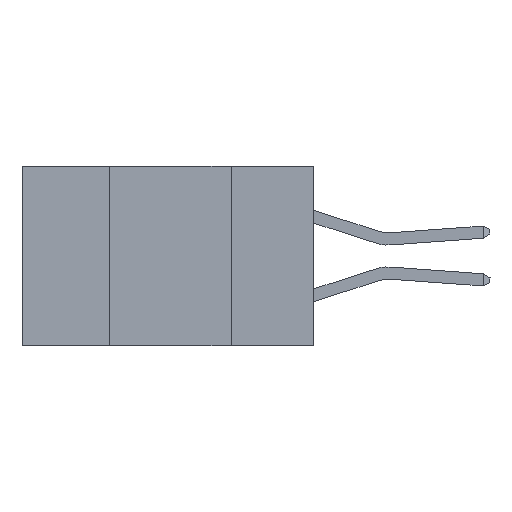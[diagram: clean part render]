
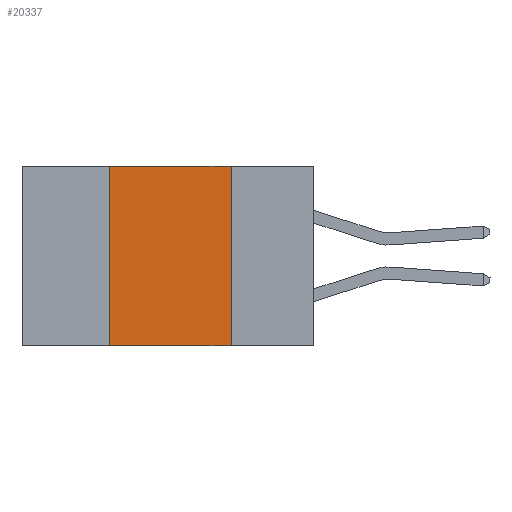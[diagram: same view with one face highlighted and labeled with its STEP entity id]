
A CAD part, left-side view. The second image highlights one B-rep face of the part: STEP entity #20337.
In plain terms, the highlighted planar face has unit normal (-1, 0, 0).
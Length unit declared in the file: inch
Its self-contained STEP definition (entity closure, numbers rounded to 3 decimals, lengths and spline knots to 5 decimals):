
#322 = VERTEX_POINT ( 'NONE', #6446 ) ;
#919 = DIRECTION ( 'NONE',  ( 0., 0., -1. ) ) ;
#938 = VECTOR ( 'NONE', #1558, 39.37008 ) ;
#1558 = DIRECTION ( 'NONE',  ( 0., -1., 0. ) ) ;
#1697 = CARTESIAN_POINT ( 'NONE',  ( 0., 0.17, 0. ) ) ;
#2396 = LINE ( 'NONE', #8140, #18424 ) ;
#3722 = ORIENTED_EDGE ( 'NONE', *, *, #6711, .F. ) ;
#3959 = CARTESIAN_POINT ( 'NONE',  ( 0., 0.42, 0. ) ) ;
#4255 = VECTOR ( 'NONE', #16908, 39.37008 ) ;
#5493 = FACE_OUTER_BOUND ( 'NONE', #22182, .T. ) ;
#5604 = CARTESIAN_POINT ( 'NONE',  ( 0., 0.17, 0. ) ) ;
#5704 = DIRECTION ( 'NONE',  ( 0., 0., -1. ) ) ;
#6232 = CARTESIAN_POINT ( 'NONE',  ( 0., 0.6, 0. ) ) ;
#6446 = CARTESIAN_POINT ( 'NONE',  ( 0., 0.17, -0.37 ) ) ;
#6711 = EDGE_CURVE ( 'NONE', #20860, #8819, #2396, .T. ) ;
#7575 = EDGE_CURVE ( 'NONE', #17373, #322, #7737, .T. ) ;
#7737 = LINE ( 'NONE', #23110, #938 ) ;
#8108 = DIRECTION ( 'NONE',  ( 1., 0., 0. ) ) ;
#8140 = CARTESIAN_POINT ( 'NONE',  ( 0., 0.6, 0. ) ) ;
#8819 = VERTEX_POINT ( 'NONE', #1697 ) ;
#9118 = EDGE_CURVE ( 'NONE', #17373, #20860, #15782, .T. ) ;
#10176 = EDGE_CURVE ( 'NONE', #8819, #322, #13766, .T. ) ;
#11070 = PLANE ( 'NONE',  #17179 ) ;
#11631 = CARTESIAN_POINT ( 'NONE',  ( 0., 0.42, -0.37 ) ) ;
#12637 = VECTOR ( 'NONE', #5704, 39.37008 ) ;
#12966 = ORIENTED_EDGE ( 'NONE', *, *, #9118, .F. ) ;
#13245 = ORIENTED_EDGE ( 'NONE', *, *, #10176, .F. ) ;
#13706 = DIRECTION ( 'NONE',  ( 0., -1., 0. ) ) ;
#13766 = LINE ( 'NONE', #5604, #12637 ) ;
#15782 = LINE ( 'NONE', #3959, #4255 ) ;
#16908 = DIRECTION ( 'NONE',  ( 0., 0., 1. ) ) ;
#17179 = AXIS2_PLACEMENT_3D ( 'NONE', #6232, #8108, #919 ) ;
#17373 = VERTEX_POINT ( 'NONE', #11631 ) ;
#18390 = ORIENTED_EDGE ( 'NONE', *, *, #7575, .T. ) ;
#18424 = VECTOR ( 'NONE', #13706, 39.37008 ) ;
#20337 = ADVANCED_FACE ( 'NONE', ( #5493 ), #11070, .F. ) ;
#20860 = VERTEX_POINT ( 'NONE', #22680 ) ;
#22182 = EDGE_LOOP ( 'NONE', ( #13245, #3722, #12966, #18390 ) ) ;
#22680 = CARTESIAN_POINT ( 'NONE',  ( 0., 0.42, 0. ) ) ;
#23110 = CARTESIAN_POINT ( 'NONE',  ( 0., 0.6, -0.37 ) ) ;
